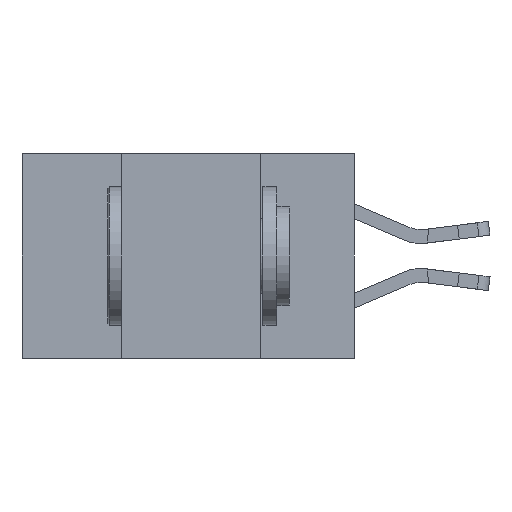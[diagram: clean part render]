
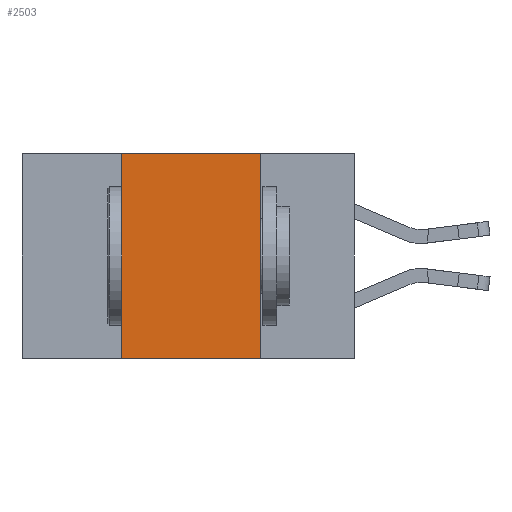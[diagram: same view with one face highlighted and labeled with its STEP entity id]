
A CAD part, left-side view. The second image highlights one B-rep face of the part: STEP entity #2503.
In plain terms, the highlighted planar face has unit normal (-1, 0, 0).
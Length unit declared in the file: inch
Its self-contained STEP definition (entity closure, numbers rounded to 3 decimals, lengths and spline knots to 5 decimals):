
#370 = EDGE_CURVE ( 'NONE', #8916, #12602, #5669, .T. ) ;
#645 = CARTESIAN_POINT ( 'NONE',  ( 0., 0.6, 0. ) ) ;
#1163 = AXIS2_PLACEMENT_3D ( 'NONE', #9433, #2019, #1833 ) ;
#1792 = CARTESIAN_POINT ( 'NONE',  ( 0., 0.42, 0. ) ) ;
#1833 = DIRECTION ( 'NONE',  ( 0., 0., -1. ) ) ;
#2019 = DIRECTION ( 'NONE',  ( 1., 0., 0. ) ) ;
#2201 = EDGE_CURVE ( 'NONE', #10043, #11880, #2567, .T. ) ;
#2269 = LINE ( 'NONE', #3982, #13216 ) ;
#2503 = ADVANCED_FACE ( 'NONE', ( #12684 ), #8410, .F. ) ;
#2567 = LINE ( 'NONE', #6707, #3725 ) ;
#3588 = EDGE_CURVE ( 'NONE', #11880, #8916, #10518, .T. ) ;
#3725 = VECTOR ( 'NONE', #10964, 39.37008 ) ;
#3982 = CARTESIAN_POINT ( 'NONE',  ( 0., 0.6, -0.37 ) ) ;
#4366 = ORIENTED_EDGE ( 'NONE', *, *, #6560, .T. ) ;
#5188 = CARTESIAN_POINT ( 'NONE',  ( 0., 0.17, 0. ) ) ;
#5669 = LINE ( 'NONE', #6837, #10662 ) ;
#5721 = DIRECTION ( 'NONE',  ( 0., 0., -1. ) ) ;
#6560 = EDGE_CURVE ( 'NONE', #10043, #12602, #2269, .T. ) ;
#6707 = CARTESIAN_POINT ( 'NONE',  ( 0., 0.42, 0. ) ) ;
#6837 = CARTESIAN_POINT ( 'NONE',  ( 0., 0.17, 0. ) ) ;
#6968 = ORIENTED_EDGE ( 'NONE', *, *, #2201, .F. ) ;
#8196 = VECTOR ( 'NONE', #9093, 39.37008 ) ;
#8410 = PLANE ( 'NONE',  #1163 ) ;
#8916 = VERTEX_POINT ( 'NONE', #5188 ) ;
#9093 = DIRECTION ( 'NONE',  ( 0., -1., 0. ) ) ;
#9433 = CARTESIAN_POINT ( 'NONE',  ( 0., 0.6, 0. ) ) ;
#9721 = ORIENTED_EDGE ( 'NONE', *, *, #370, .F. ) ;
#10043 = VERTEX_POINT ( 'NONE', #13069 ) ;
#10257 = DIRECTION ( 'NONE',  ( 0., -1., 0. ) ) ;
#10518 = LINE ( 'NONE', #645, #8196 ) ;
#10662 = VECTOR ( 'NONE', #5721, 39.37008 ) ;
#10964 = DIRECTION ( 'NONE',  ( 0., 0., 1. ) ) ;
#11653 = CARTESIAN_POINT ( 'NONE',  ( 0., 0.17, -0.37 ) ) ;
#11880 = VERTEX_POINT ( 'NONE', #1792 ) ;
#11883 = ORIENTED_EDGE ( 'NONE', *, *, #3588, .F. ) ;
#12400 = EDGE_LOOP ( 'NONE', ( #9721, #11883, #6968, #4366 ) ) ;
#12602 = VERTEX_POINT ( 'NONE', #11653 ) ;
#12684 = FACE_OUTER_BOUND ( 'NONE', #12400, .T. ) ;
#13069 = CARTESIAN_POINT ( 'NONE',  ( 0., 0.42, -0.37 ) ) ;
#13216 = VECTOR ( 'NONE', #10257, 39.37008 ) ;
